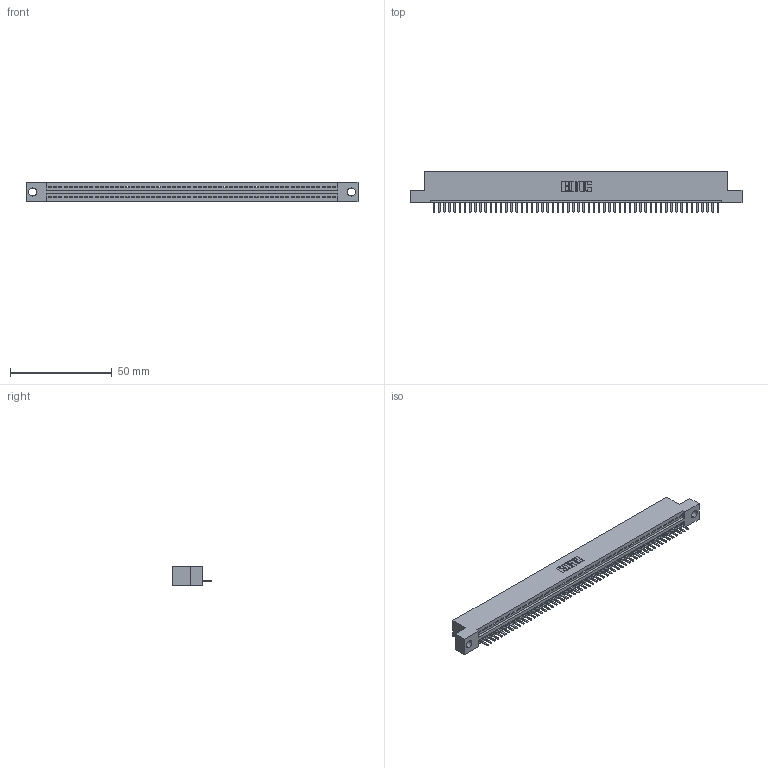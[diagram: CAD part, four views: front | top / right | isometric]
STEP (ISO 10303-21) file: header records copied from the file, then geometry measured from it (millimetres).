
FILE_DESCRIPTION (( 'STEP AP203' ), '1' );
FILE_NAME ('345-056-520-104.STEP', '2021-05-28T15:36:22', ( '' ), ( '' ), 'SwSTEP 2.0', 'SolidWorks 2020', '' );
FILE_SCHEMA (( 'CONFIG_CONTROL_DESIGN' ));
Length unit declared in the file: inch
Products named in the file (3): 345 Part_Flush Mounting Lugs - 0.156 Dia-TI; 345-056-520-104; 345-292-001_345-293-120
Assembly tree (57 placements, depth 2):
  345-056-520-104
    345 Part_Flush Mounting Lugs - 0.156 Dia-TI
    345-292-001_345-293-120  x56
Bounding box: 163.45 x 19.68 x 9.4 mm (x, y, z)
Volume: 15372.2 mm3; surface area: 19934 mm2
Topology: 57 solids, 57 shells, 3612 faces, 10681 edges, 6970 vertices
Faces by surface type: plane 2446, cylinder 1166
Entity records: 40795 total; most frequent: CARTESIAN_POINT 7086, ORIENTED_EDGE 7062, DIRECTION 6155, EDGE_CURVE 3531, LINE 3171, VECTOR 3171, VERTEX_POINT 2350, AXIS2_PLACEMENT_3D 1492
